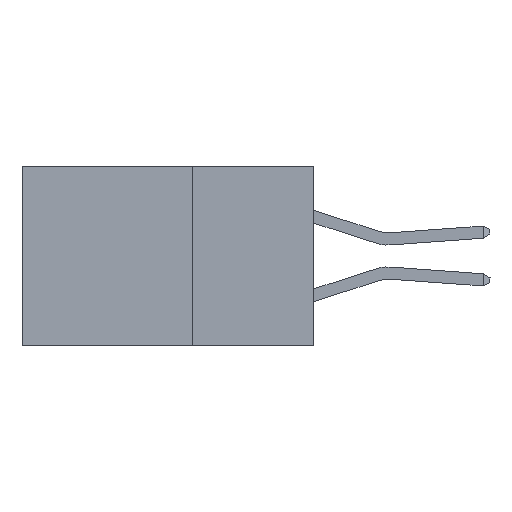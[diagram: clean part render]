
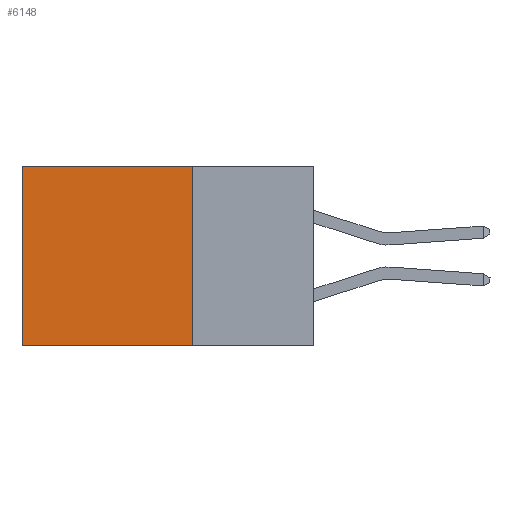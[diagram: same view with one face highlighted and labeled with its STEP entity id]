
A CAD part, left-side view. The second image highlights one B-rep face of the part: STEP entity #6148.
In plain terms, the highlighted planar face has unit normal (-1, 0, 0).
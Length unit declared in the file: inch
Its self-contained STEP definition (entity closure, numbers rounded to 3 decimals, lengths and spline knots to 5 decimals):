
#284 = VECTOR ( 'NONE', #12930, 39.37008 ) ;
#1283 = DIRECTION ( 'NONE',  ( 0., 1., 0. ) ) ;
#1947 = EDGE_CURVE ( 'NONE', #8408, #21801, #10554, .T. ) ;
#2363 = EDGE_CURVE ( 'NONE', #12277, #21186, #20880, .T. ) ;
#2717 = AXIS2_PLACEMENT_3D ( 'NONE', #24681, #14993, #18758 ) ;
#5863 = CARTESIAN_POINT ( 'NONE',  ( 0.2875, 0.25, 0. ) ) ;
#6148 = ADVANCED_FACE ( 'NONE', ( #12901 ), #22699, .F. ) ;
#8408 = VERTEX_POINT ( 'NONE', #5863 ) ;
#8496 = ORIENTED_EDGE ( 'NONE', *, *, #19762, .F. ) ;
#8613 = ORIENTED_EDGE ( 'NONE', *, *, #2363, .T. ) ;
#8801 = CARTESIAN_POINT ( 'NONE',  ( 0.2875, 0.6, 0. ) ) ;
#9084 = CARTESIAN_POINT ( 'NONE',  ( 0.2875, 0.25, -0.37 ) ) ;
#10554 = LINE ( 'NONE', #21519, #19663 ) ;
#11457 = CARTESIAN_POINT ( 'NONE',  ( 0.2875, 0.6, -0.37 ) ) ;
#11920 = LINE ( 'NONE', #21505, #21021 ) ;
#12216 = CARTESIAN_POINT ( 'NONE',  ( 0.2875, 0.25, -0.37 ) ) ;
#12277 = VERTEX_POINT ( 'NONE', #13514 ) ;
#12901 = FACE_OUTER_BOUND ( 'NONE', #23538, .T. ) ;
#12930 = DIRECTION ( 'NONE',  ( 0., 1., 0. ) ) ;
#13514 = CARTESIAN_POINT ( 'NONE',  ( 0.2875, 0.6, 0. ) ) ;
#13652 = DIRECTION ( 'NONE',  ( 0., 0., -1. ) ) ;
#14993 = DIRECTION ( 'NONE',  ( 1., 0., 0. ) ) ;
#15077 = DIRECTION ( 'NONE',  ( 0., 0., -1. ) ) ;
#15601 = ORIENTED_EDGE ( 'NONE', *, *, #17882, .T. ) ;
#17882 = EDGE_CURVE ( 'NONE', #8408, #12277, #11920, .T. ) ;
#18360 = VECTOR ( 'NONE', #15077, 39.37008 ) ;
#18758 = DIRECTION ( 'NONE',  ( 0., 0., -1. ) ) ;
#19663 = VECTOR ( 'NONE', #13652, 39.37008 ) ;
#19762 = EDGE_CURVE ( 'NONE', #21801, #21186, #24889, .T. ) ;
#20880 = LINE ( 'NONE', #8801, #18360 ) ;
#21021 = VECTOR ( 'NONE', #1283, 39.37008 ) ;
#21186 = VERTEX_POINT ( 'NONE', #11457 ) ;
#21505 = CARTESIAN_POINT ( 'NONE',  ( 0.2875, 0.25, 0. ) ) ;
#21519 = CARTESIAN_POINT ( 'NONE',  ( 0.2875, 0.25, 0. ) ) ;
#21801 = VERTEX_POINT ( 'NONE', #12216 ) ;
#22699 = PLANE ( 'NONE',  #2717 ) ;
#23538 = EDGE_LOOP ( 'NONE', ( #8613, #8496, #25254, #15601 ) ) ;
#24681 = CARTESIAN_POINT ( 'NONE',  ( 0.2875, 0.25, 0. ) ) ;
#24889 = LINE ( 'NONE', #9084, #284 ) ;
#25254 = ORIENTED_EDGE ( 'NONE', *, *, #1947, .F. ) ;
